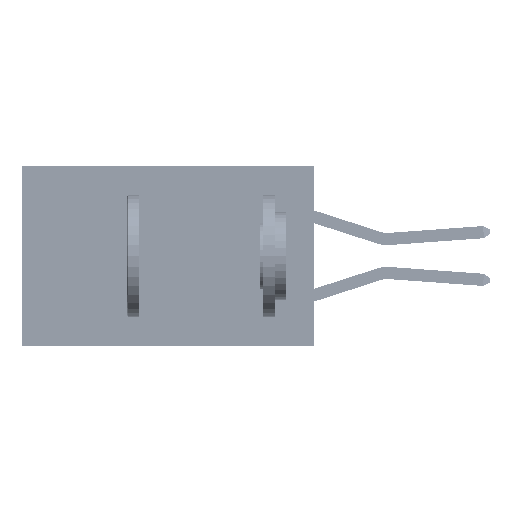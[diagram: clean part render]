
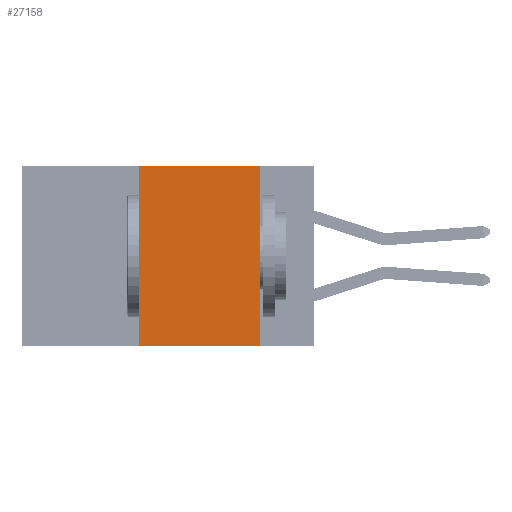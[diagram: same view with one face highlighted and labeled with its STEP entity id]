
A CAD part, left-side view. The second image highlights one B-rep face of the part: STEP entity #27158.
In plain terms, the highlighted planar face has unit normal (-1, 0, 0).
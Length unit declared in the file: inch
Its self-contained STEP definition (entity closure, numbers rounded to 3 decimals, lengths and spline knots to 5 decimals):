
#1655 = VECTOR ( 'NONE', #22092, 39.37008 ) ;
#4785 = VECTOR ( 'NONE', #28543, 39.37008 ) ;
#6331 = EDGE_CURVE ( 'NONE', #24303, #17184, #15766, .T. ) ;
#6661 = ORIENTED_EDGE ( 'NONE', *, *, #20406, .F. ) ;
#7612 = CARTESIAN_POINT ( 'NONE',  ( 0., 0.36, 0. ) ) ;
#13147 = CARTESIAN_POINT ( 'NONE',  ( 0., 0.11, -0.37 ) ) ;
#14065 = CARTESIAN_POINT ( 'NONE',  ( 0., 0.11, 0. ) ) ;
#15766 = LINE ( 'NONE', #37086, #19874 ) ;
#17007 = DIRECTION ( 'NONE',  ( 0., -1., 0. ) ) ;
#17184 = VERTEX_POINT ( 'NONE', #45840 ) ;
#18164 = LINE ( 'NONE', #7612, #1655 ) ;
#18842 = CARTESIAN_POINT ( 'NONE',  ( 0., 0.36, -0.37 ) ) ;
#19790 = EDGE_LOOP ( 'NONE', ( #22589, #26366, #6661, #47775 ) ) ;
#19874 = VECTOR ( 'NONE', #17007, 39.37008 ) ;
#20162 = LINE ( 'NONE', #14065, #4785 ) ;
#20406 = EDGE_CURVE ( 'NONE', #26193, #24303, #18164, .T. ) ;
#20708 = DIRECTION ( 'NONE',  ( 0., -1., 0. ) ) ;
#21137 = CARTESIAN_POINT ( 'NONE',  ( 0., 0.6, 0. ) ) ;
#22092 = DIRECTION ( 'NONE',  ( 0., 0., 1. ) ) ;
#22488 = AXIS2_PLACEMENT_3D ( 'NONE', #21137, #40219, #32484 ) ;
#22589 = ORIENTED_EDGE ( 'NONE', *, *, #27072, .F. ) ;
#24147 = CARTESIAN_POINT ( 'NONE',  ( 0., 0.6, -0.37 ) ) ;
#24303 = VERTEX_POINT ( 'NONE', #26220 ) ;
#26193 = VERTEX_POINT ( 'NONE', #18842 ) ;
#26220 = CARTESIAN_POINT ( 'NONE',  ( 0., 0.36, 0. ) ) ;
#26366 = ORIENTED_EDGE ( 'NONE', *, *, #6331, .F. ) ;
#27072 = EDGE_CURVE ( 'NONE', #17184, #29090, #20162, .T. ) ;
#27158 = ADVANCED_FACE ( 'NONE', ( #27236 ), #36119, .F. ) ;
#27236 = FACE_OUTER_BOUND ( 'NONE', #19790, .T. ) ;
#28543 = DIRECTION ( 'NONE',  ( 0., 0., -1. ) ) ;
#29090 = VERTEX_POINT ( 'NONE', #13147 ) ;
#30376 = VECTOR ( 'NONE', #20708, 39.37008 ) ;
#31667 = EDGE_CURVE ( 'NONE', #26193, #29090, #36269, .T. ) ;
#32484 = DIRECTION ( 'NONE',  ( 0., 0., -1. ) ) ;
#36119 = PLANE ( 'NONE',  #22488 ) ;
#36269 = LINE ( 'NONE', #24147, #30376 ) ;
#37086 = CARTESIAN_POINT ( 'NONE',  ( 0., 0.6, 0. ) ) ;
#40219 = DIRECTION ( 'NONE',  ( 1., 0., 0. ) ) ;
#45840 = CARTESIAN_POINT ( 'NONE',  ( 0., 0.11, 0. ) ) ;
#47775 = ORIENTED_EDGE ( 'NONE', *, *, #31667, .T. ) ;
